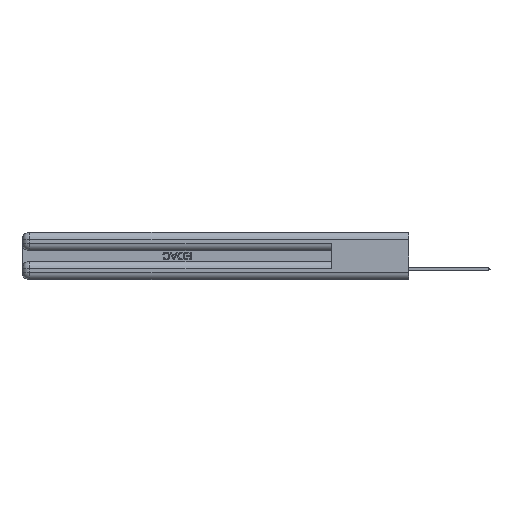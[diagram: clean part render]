
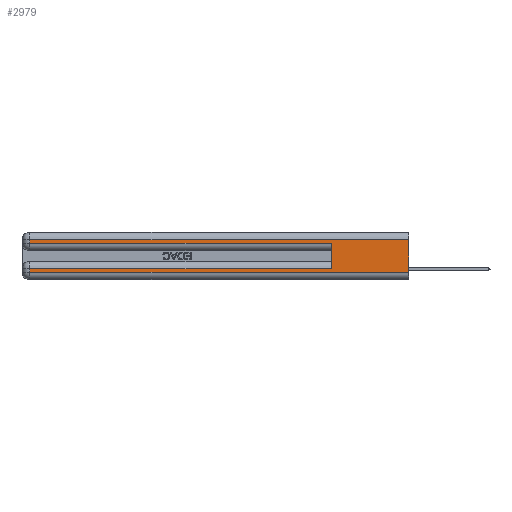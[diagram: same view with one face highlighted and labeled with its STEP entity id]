
A CAD part, left-side view. The second image highlights one B-rep face of the part: STEP entity #2979.
In plain terms, the highlighted planar face has unit normal (-1, 0, 0).
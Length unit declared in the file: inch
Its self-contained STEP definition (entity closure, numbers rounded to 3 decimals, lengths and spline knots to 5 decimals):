
#641 = VERTEX_POINT ( 'NONE', #2960 ) ;
#1036 = CARTESIAN_POINT ( 'NONE',  ( 0., 0., 0.06 ) ) ;
#2306 = CARTESIAN_POINT ( 'NONE',  ( 0., 2.94, 0.285 ) ) ;
#2960 = CARTESIAN_POINT ( 'NONE',  ( 0., 0.6, 0.085 ) ) ;
#2979 = ADVANCED_FACE ( 'NONE', ( #40109 ), #14020, .F. ) ;
#3923 = ORIENTED_EDGE ( 'NONE', *, *, #47815, .F. ) ;
#4136 = EDGE_LOOP ( 'NONE', ( #25109, #25083, #23876, #13064, #3923, #12921, #47476, #29657 ) ) ;
#5057 = CARTESIAN_POINT ( 'NONE',  ( 0., 2.94, 0.085 ) ) ;
#5222 = VECTOR ( 'NONE', #18297, 39.37008 ) ;
#5468 = VERTEX_POINT ( 'NONE', #2306 ) ;
#6355 = CARTESIAN_POINT ( 'NONE',  ( 0., 0., 0.31 ) ) ;
#10209 = CARTESIAN_POINT ( 'NONE',  ( 0., 0.6, 0.285 ) ) ;
#10981 = VERTEX_POINT ( 'NONE', #6355 ) ;
#11886 = CARTESIAN_POINT ( 'NONE',  ( 0., 0., 0.085 ) ) ;
#12044 = DIRECTION ( 'NONE',  ( 0., 1., 0. ) ) ;
#12774 = DIRECTION ( 'NONE',  ( 0., 1., 0. ) ) ;
#12921 = ORIENTED_EDGE ( 'NONE', *, *, #31829, .T. ) ;
#13064 = ORIENTED_EDGE ( 'NONE', *, *, #16860, .T. ) ;
#13591 = DIRECTION ( 'NONE',  ( 0., 0., -1. ) ) ;
#14020 = PLANE ( 'NONE',  #26926 ) ;
#15732 = VECTOR ( 'NONE', #23909, 39.37008 ) ;
#16006 = VERTEX_POINT ( 'NONE', #5057 ) ;
#16121 = VECTOR ( 'NONE', #47691, 39.37008 ) ;
#16152 = LINE ( 'NONE', #11886, #19743 ) ;
#16860 = EDGE_CURVE ( 'NONE', #5468, #45002, #37247, .T. ) ;
#18297 = DIRECTION ( 'NONE',  ( 0., 0., -1. ) ) ;
#19656 = VERTEX_POINT ( 'NONE', #36585 ) ;
#19743 = VECTOR ( 'NONE', #12044, 39.37008 ) ;
#21694 = DIRECTION ( 'NONE',  ( 0., 0., -1. ) ) ;
#22960 = EDGE_CURVE ( 'NONE', #10981, #33168, #25973, .T. ) ;
#23464 = VERTEX_POINT ( 'NONE', #30862 ) ;
#23876 = ORIENTED_EDGE ( 'NONE', *, *, #38402, .T. ) ;
#23909 = DIRECTION ( 'NONE',  ( 0., -1., 0. ) ) ;
#24648 = EDGE_CURVE ( 'NONE', #10981, #23464, #44379, .T. ) ;
#25083 = ORIENTED_EDGE ( 'NONE', *, *, #24648, .T. ) ;
#25109 = ORIENTED_EDGE ( 'NONE', *, *, #22960, .F. ) ;
#25973 = LINE ( 'NONE', #34192, #31235 ) ;
#26926 = AXIS2_PLACEMENT_3D ( 'NONE', #32783, #36486, #21694 ) ;
#28136 = VECTOR ( 'NONE', #34749, 39.37008 ) ;
#28565 = EDGE_CURVE ( 'NONE', #16006, #19656, #38647, .T. ) ;
#28754 = CARTESIAN_POINT ( 'NONE',  ( 0., 0.6, 0.145 ) ) ;
#29657 = ORIENTED_EDGE ( 'NONE', *, *, #46435, .T. ) ;
#30862 = CARTESIAN_POINT ( 'NONE',  ( 0., 2.94, 0.31 ) ) ;
#31007 = CARTESIAN_POINT ( 'NONE',  ( 0., 0., 0.31 ) ) ;
#31235 = VECTOR ( 'NONE', #44462, 39.37008 ) ;
#31829 = EDGE_CURVE ( 'NONE', #641, #16006, #16152, .T. ) ;
#32783 = CARTESIAN_POINT ( 'NONE',  ( 0., 0., 0.37 ) ) ;
#33168 = VERTEX_POINT ( 'NONE', #34696 ) ;
#33771 = CARTESIAN_POINT ( 'NONE',  ( 0., 2.94, 0.37 ) ) ;
#34192 = CARTESIAN_POINT ( 'NONE',  ( 0., 0., 0.37 ) ) ;
#34299 = LINE ( 'NONE', #37293, #5222 ) ;
#34696 = CARTESIAN_POINT ( 'NONE',  ( 0., 0., 0.06 ) ) ;
#34749 = DIRECTION ( 'NONE',  ( 0., -1., 0. ) ) ;
#35219 = CARTESIAN_POINT ( 'NONE',  ( 0., 0., 0.285 ) ) ;
#36486 = DIRECTION ( 'NONE',  ( 1., 0., 0. ) ) ;
#36585 = CARTESIAN_POINT ( 'NONE',  ( 0., 2.94, 0.06 ) ) ;
#37247 = LINE ( 'NONE', #35219, #15732 ) ;
#37293 = CARTESIAN_POINT ( 'NONE',  ( 0., 2.94, 0.37 ) ) ;
#37551 = VECTOR ( 'NONE', #13591, 39.37008 ) ;
#37871 = VECTOR ( 'NONE', #12774, 39.37008 ) ;
#38402 = EDGE_CURVE ( 'NONE', #23464, #5468, #34299, .T. ) ;
#38647 = LINE ( 'NONE', #33771, #37551 ) ;
#38872 = LINE ( 'NONE', #1036, #28136 ) ;
#40109 = FACE_OUTER_BOUND ( 'NONE', #4136, .T. ) ;
#44379 = LINE ( 'NONE', #31007, #37871 ) ;
#44462 = DIRECTION ( 'NONE',  ( 0., 0., -1. ) ) ;
#45002 = VERTEX_POINT ( 'NONE', #10209 ) ;
#46435 = EDGE_CURVE ( 'NONE', #19656, #33168, #38872, .T. ) ;
#47004 = LINE ( 'NONE', #28754, #16121 ) ;
#47476 = ORIENTED_EDGE ( 'NONE', *, *, #28565, .T. ) ;
#47691 = DIRECTION ( 'NONE',  ( 0., 0., 1. ) ) ;
#47815 = EDGE_CURVE ( 'NONE', #641, #45002, #47004, .T. ) ;
